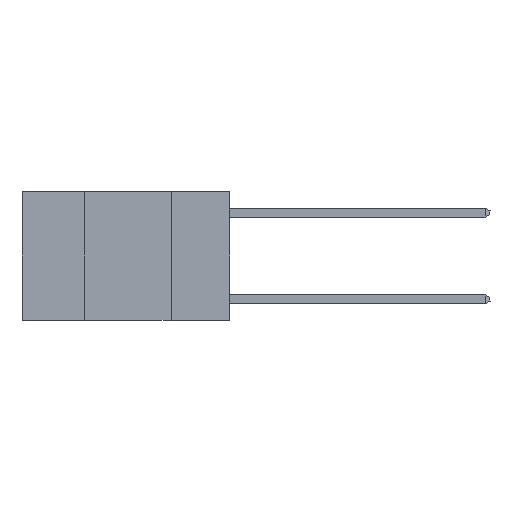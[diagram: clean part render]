
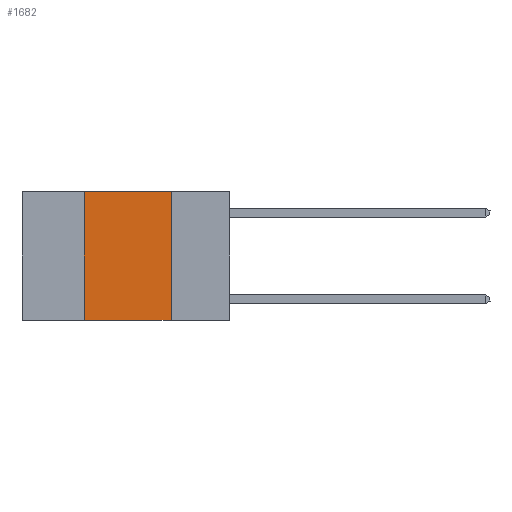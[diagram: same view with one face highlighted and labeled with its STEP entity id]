
A CAD part, left-side view. The second image highlights one B-rep face of the part: STEP entity #1682.
In plain terms, the highlighted planar face has unit normal (-1, 0, 0).
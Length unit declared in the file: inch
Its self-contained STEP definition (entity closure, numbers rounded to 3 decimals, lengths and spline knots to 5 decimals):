
#113 = ORIENTED_EDGE ( 'NONE', *, *, #25029, .T. ) ;
#257 = EDGE_CURVE ( 'NONE', #1028, #27866, #5412, .T. ) ;
#820 = CARTESIAN_POINT ( 'NONE',  ( 0., 0.17, 0. ) ) ;
#1028 = VERTEX_POINT ( 'NONE', #1640 ) ;
#1640 = CARTESIAN_POINT ( 'NONE',  ( 0., 0.42, -0.37 ) ) ;
#1682 = ADVANCED_FACE ( 'NONE', ( #3569 ), #8318, .F. ) ;
#3569 = FACE_OUTER_BOUND ( 'NONE', #22693, .T. ) ;
#3628 = VECTOR ( 'NONE', #30144, 39.37008 ) ;
#3717 = AXIS2_PLACEMENT_3D ( 'NONE', #7721, #24464, #15212 ) ;
#4538 = VECTOR ( 'NONE', #22201, 39.37008 ) ;
#5412 = LINE ( 'NONE', #8015, #26177 ) ;
#5805 = CARTESIAN_POINT ( 'NONE',  ( 0., 0.42, 0. ) ) ;
#6635 = LINE ( 'NONE', #7084, #3628 ) ;
#7084 = CARTESIAN_POINT ( 'NONE',  ( 0., 0.6, 0. ) ) ;
#7721 = CARTESIAN_POINT ( 'NONE',  ( 0., 0.6, 0. ) ) ;
#8015 = CARTESIAN_POINT ( 'NONE',  ( 0., 0.42, 0. ) ) ;
#8318 = PLANE ( 'NONE',  #3717 ) ;
#8790 = EDGE_CURVE ( 'NONE', #11172, #12930, #19701, .T. ) ;
#9126 = CARTESIAN_POINT ( 'NONE',  ( 0., 0.17, -0.37 ) ) ;
#9380 = ORIENTED_EDGE ( 'NONE', *, *, #8790, .F. ) ;
#10951 = ORIENTED_EDGE ( 'NONE', *, *, #27145, .F. ) ;
#11172 = VERTEX_POINT ( 'NONE', #20238 ) ;
#12930 = VERTEX_POINT ( 'NONE', #9126 ) ;
#14759 = DIRECTION ( 'NONE',  ( 0., 0., 1. ) ) ;
#15212 = DIRECTION ( 'NONE',  ( 0., 0., -1. ) ) ;
#16841 = VECTOR ( 'NONE', #19847, 39.37008 ) ;
#17877 = CARTESIAN_POINT ( 'NONE',  ( 0., 0.6, -0.37 ) ) ;
#19701 = LINE ( 'NONE', #820, #16841 ) ;
#19847 = DIRECTION ( 'NONE',  ( 0., 0., -1. ) ) ;
#20238 = CARTESIAN_POINT ( 'NONE',  ( 0., 0.17, 0. ) ) ;
#22201 = DIRECTION ( 'NONE',  ( 0., -1., 0. ) ) ;
#22693 = EDGE_LOOP ( 'NONE', ( #9380, #10951, #25910, #113 ) ) ;
#24464 = DIRECTION ( 'NONE',  ( 1., 0., 0. ) ) ;
#25029 = EDGE_CURVE ( 'NONE', #1028, #12930, #27448, .T. ) ;
#25910 = ORIENTED_EDGE ( 'NONE', *, *, #257, .F. ) ;
#26177 = VECTOR ( 'NONE', #14759, 39.37008 ) ;
#27145 = EDGE_CURVE ( 'NONE', #27866, #11172, #6635, .T. ) ;
#27448 = LINE ( 'NONE', #17877, #4538 ) ;
#27866 = VERTEX_POINT ( 'NONE', #5805 ) ;
#30144 = DIRECTION ( 'NONE',  ( 0., -1., 0. ) ) ;
